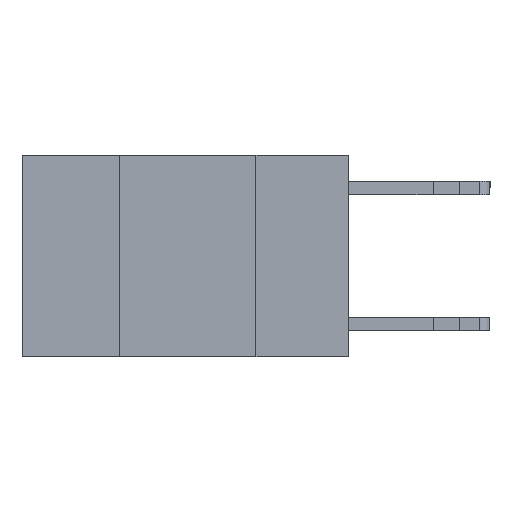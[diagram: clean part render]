
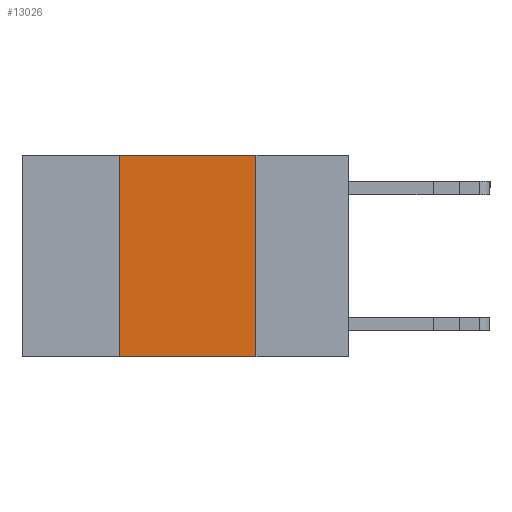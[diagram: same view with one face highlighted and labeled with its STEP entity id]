
A CAD part, left-side view. The second image highlights one B-rep face of the part: STEP entity #13026.
In plain terms, the highlighted planar face has unit normal (-1, 0, 0).
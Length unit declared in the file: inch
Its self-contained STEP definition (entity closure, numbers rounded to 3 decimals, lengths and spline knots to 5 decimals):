
#41 = VERTEX_POINT ( 'NONE', #13402 ) ;
#517 = AXIS2_PLACEMENT_3D ( 'NONE', #8760, #13310, #15229 ) ;
#685 = CARTESIAN_POINT ( 'NONE',  ( 0., 0.42, -0.37 ) ) ;
#1100 = VECTOR ( 'NONE', #19886, 39.37008 ) ;
#2005 = DIRECTION ( 'NONE',  ( 0., 0., 1. ) ) ;
#2426 = LINE ( 'NONE', #13417, #1100 ) ;
#3385 = ORIENTED_EDGE ( 'NONE', *, *, #12859, .F. ) ;
#3854 = VERTEX_POINT ( 'NONE', #685 ) ;
#4614 = VECTOR ( 'NONE', #19422, 39.37008 ) ;
#4876 = VECTOR ( 'NONE', #18075, 39.37008 ) ;
#5162 = CARTESIAN_POINT ( 'NONE',  ( 0., 0.17, 0. ) ) ;
#6329 = EDGE_CURVE ( 'NONE', #3854, #41, #2426, .T. ) ;
#7401 = VERTEX_POINT ( 'NONE', #14808 ) ;
#7650 = CARTESIAN_POINT ( 'NONE',  ( 0., 0.17, 0. ) ) ;
#8760 = CARTESIAN_POINT ( 'NONE',  ( 0., 0.6, 0. ) ) ;
#9552 = EDGE_LOOP ( 'NONE', ( #10231, #20230, #3385, #16936 ) ) ;
#10231 = ORIENTED_EDGE ( 'NONE', *, *, #12931, .F. ) ;
#11628 = CARTESIAN_POINT ( 'NONE',  ( 0., 0.42, 0. ) ) ;
#12859 = EDGE_CURVE ( 'NONE', #3854, #7401, #16170, .T. ) ;
#12931 = EDGE_CURVE ( 'NONE', #17363, #41, #19239, .T. ) ;
#12968 = LINE ( 'NONE', #17835, #4614 ) ;
#13026 = ADVANCED_FACE ( 'NONE', ( #16798 ), #13514, .F. ) ;
#13310 = DIRECTION ( 'NONE',  ( 1., 0., 0. ) ) ;
#13402 = CARTESIAN_POINT ( 'NONE',  ( 0., 0.17, -0.37 ) ) ;
#13417 = CARTESIAN_POINT ( 'NONE',  ( 0., 0.6, -0.37 ) ) ;
#13514 = PLANE ( 'NONE',  #517 ) ;
#14808 = CARTESIAN_POINT ( 'NONE',  ( 0., 0.42, 0. ) ) ;
#15229 = DIRECTION ( 'NONE',  ( 0., 0., -1. ) ) ;
#16170 = LINE ( 'NONE', #11628, #19419 ) ;
#16798 = FACE_OUTER_BOUND ( 'NONE', #9552, .T. ) ;
#16936 = ORIENTED_EDGE ( 'NONE', *, *, #6329, .T. ) ;
#17153 = EDGE_CURVE ( 'NONE', #7401, #17363, #12968, .T. ) ;
#17363 = VERTEX_POINT ( 'NONE', #7650 ) ;
#17835 = CARTESIAN_POINT ( 'NONE',  ( 0., 0.6, 0. ) ) ;
#18075 = DIRECTION ( 'NONE',  ( 0., 0., -1. ) ) ;
#19239 = LINE ( 'NONE', #5162, #4876 ) ;
#19419 = VECTOR ( 'NONE', #2005, 39.37008 ) ;
#19422 = DIRECTION ( 'NONE',  ( 0., -1., 0. ) ) ;
#19886 = DIRECTION ( 'NONE',  ( 0., -1., 0. ) ) ;
#20230 = ORIENTED_EDGE ( 'NONE', *, *, #17153, .F. ) ;
